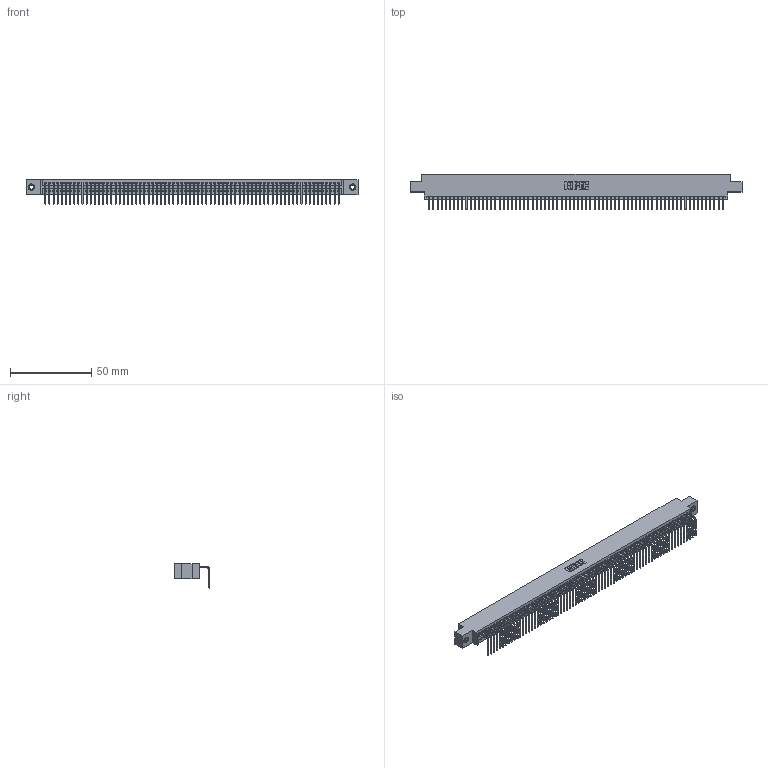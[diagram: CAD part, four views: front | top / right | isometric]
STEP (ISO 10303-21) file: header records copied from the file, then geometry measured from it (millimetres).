
FILE_DESCRIPTION (( 'STEP AP203' ), '1' );
FILE_NAME ('395-072-558-607.STEP', '2018-11-27T15:56:42', ( '' ), ( '' ), 'SwSTEP 2.0', 'SolidWorks 2016', '' );
FILE_SCHEMA (( 'CONFIG_CONTROL_DESIGN' ));
Length unit declared in the file: inch
Products named in the file (4): 345-292-001_558 Tail - 2; 345-250-001_345-250-005-103; 345 Part_0.170 Offset - 0.156 Dia-TI; 395-072-558-607
Assembly tree (75 placements, depth 2):
  395-072-558-607
    345 Part_0.170 Offset - 0.156 Dia-TI
    345-292-001_558 Tail - 2  x72
    345-250-001_345-250-005-103  x2
Bounding box: 204.09 x 21.83 x 15.37 mm (x, y, z)
Volume: 19743.3 mm3; surface area: 28213.5 mm2
Topology: 75 solids, 75 shells, 4510 faces, 13593 edges, 8958 vertices
Faces by surface type: plane 3140, cylinder 1354, cone 12, torus 4
Entity records: 51552 total; most frequent: CARTESIAN_POINT 8911, ORIENTED_EDGE 8910, DIRECTION 7765, EDGE_CURVE 4455, VECTOR 4015, LINE 4015, VERTEX_POINT 2964, AXIS2_PLACEMENT_3D 1875
